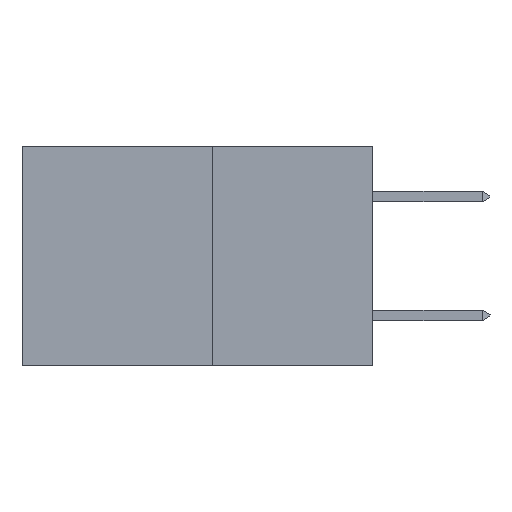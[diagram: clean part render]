
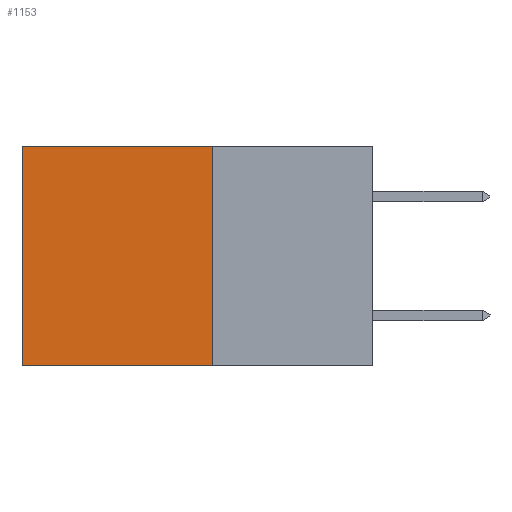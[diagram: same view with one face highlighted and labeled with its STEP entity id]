
A CAD part, left-side view. The second image highlights one B-rep face of the part: STEP entity #1153.
In plain terms, the highlighted planar face has unit normal (-1, 0, 0).
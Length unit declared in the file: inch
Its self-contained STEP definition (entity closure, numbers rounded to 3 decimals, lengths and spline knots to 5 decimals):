
#920 = VERTEX_POINT ( 'NONE', #3147 ) ;
#1091 = LINE ( 'NONE', #1880, #20946 ) ;
#1153 = ADVANCED_FACE ( 'NONE', ( #14400 ), #9337, .F. ) ;
#1880 = CARTESIAN_POINT ( 'NONE',  ( 0.277, 0.27, -0.37 ) ) ;
#3147 = CARTESIAN_POINT ( 'NONE',  ( 0.277, 0.59, 0. ) ) ;
#3503 = EDGE_CURVE ( 'NONE', #10631, #8592, #18057, .T. ) ;
#4250 = EDGE_CURVE ( 'NONE', #8592, #20342, #1091, .T. ) ;
#5745 = EDGE_CURVE ( 'NONE', #10631, #920, #18859, .T. ) ;
#5794 = CARTESIAN_POINT ( 'NONE',  ( 0.277, 0.59, -0.37 ) ) ;
#7009 = DIRECTION ( 'NONE',  ( 0., 0., -1. ) ) ;
#7050 = DIRECTION ( 'NONE',  ( 1., 0., 0. ) ) ;
#7635 = CARTESIAN_POINT ( 'NONE',  ( 0.277, 0.27, -0.37 ) ) ;
#7811 = EDGE_CURVE ( 'NONE', #920, #20342, #21114, .T. ) ;
#8187 = VECTOR ( 'NONE', #18282, 39.37008 ) ;
#8592 = VERTEX_POINT ( 'NONE', #7635 ) ;
#9337 = PLANE ( 'NONE',  #22158 ) ;
#10631 = VERTEX_POINT ( 'NONE', #20791 ) ;
#10682 = VECTOR ( 'NONE', #12478, 39.37008 ) ;
#11739 = ORIENTED_EDGE ( 'NONE', *, *, #4250, .F. ) ;
#11959 = CARTESIAN_POINT ( 'NONE',  ( 0.277, 0.59, -0.37 ) ) ;
#11995 = ORIENTED_EDGE ( 'NONE', *, *, #5745, .T. ) ;
#12478 = DIRECTION ( 'NONE',  ( 0., 0., -1. ) ) ;
#13638 = CARTESIAN_POINT ( 'NONE',  ( 0.277, 0.27, 0. ) ) ;
#13825 = DIRECTION ( 'NONE',  ( 0., 1., 0. ) ) ;
#14400 = FACE_OUTER_BOUND ( 'NONE', #21983, .T. ) ;
#16911 = CARTESIAN_POINT ( 'NONE',  ( 0.277, 0.27, -0.37 ) ) ;
#17967 = DIRECTION ( 'NONE',  ( 0., 1., 0. ) ) ;
#18057 = LINE ( 'NONE', #16911, #8187 ) ;
#18282 = DIRECTION ( 'NONE',  ( 0., 0., -1. ) ) ;
#18859 = LINE ( 'NONE', #13638, #23183 ) ;
#20342 = VERTEX_POINT ( 'NONE', #5794 ) ;
#20614 = ORIENTED_EDGE ( 'NONE', *, *, #7811, .T. ) ;
#20791 = CARTESIAN_POINT ( 'NONE',  ( 0.277, 0.27, 0. ) ) ;
#20946 = VECTOR ( 'NONE', #17967, 39.37008 ) ;
#21114 = LINE ( 'NONE', #11959, #10682 ) ;
#21983 = EDGE_LOOP ( 'NONE', ( #20614, #11739, #23682, #11995 ) ) ;
#22158 = AXIS2_PLACEMENT_3D ( 'NONE', #22850, #7050, #7009 ) ;
#22850 = CARTESIAN_POINT ( 'NONE',  ( 0.277, 0.27, -0.37 ) ) ;
#23183 = VECTOR ( 'NONE', #13825, 39.37008 ) ;
#23682 = ORIENTED_EDGE ( 'NONE', *, *, #3503, .F. ) ;
